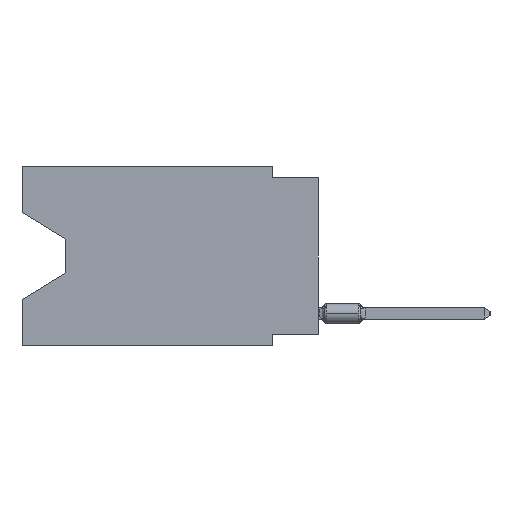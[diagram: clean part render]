
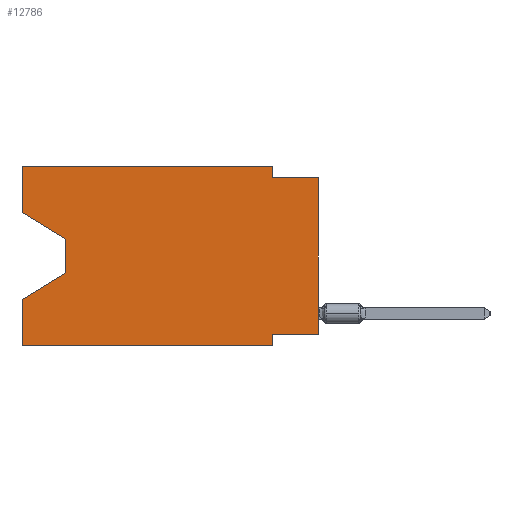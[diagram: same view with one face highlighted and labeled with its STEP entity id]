
A CAD part, left-side view. The second image highlights one B-rep face of the part: STEP entity #12786.
In plain terms, the highlighted planar face has unit normal (-1, 0, 0).
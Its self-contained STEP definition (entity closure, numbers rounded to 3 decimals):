
#658 = CARTESIAN_POINT ( 'NONE',  ( 0., 16.383, -2.546 ) ) ;
#814 = VERTEX_POINT ( 'NONE', #5526 ) ;
#831 = VERTEX_POINT ( 'NONE', #15682 ) ;
#1392 = EDGE_CURVE ( 'NONE', #14095, #26690, #18622, .T. ) ;
#1428 = EDGE_CURVE ( 'NONE', #23156, #831, #18884, .T. ) ;
#1508 = PLANE ( 'NONE',  #12656 ) ;
#3536 = CARTESIAN_POINT ( 'NONE',  ( 0., 2.54, 0. ) ) ;
#4026 = CARTESIAN_POINT ( 'NONE',  ( 0., 16.383, -2.546 ) ) ;
#4365 = ORIENTED_EDGE ( 'NONE', *, *, #9238, .F. ) ;
#4608 = ORIENTED_EDGE ( 'NONE', *, *, #15362, .F. ) ;
#4651 = EDGE_CURVE ( 'NONE', #23824, #18407, #12228, .T. ) ;
#4739 = DIRECTION ( 'NONE',  ( 0., 1., 0. ) ) ;
#4942 = ORIENTED_EDGE ( 'NONE', *, *, #26467, .T. ) ;
#5325 = VECTOR ( 'NONE', #8825, 1000. ) ;
#5526 = CARTESIAN_POINT ( 'NONE',  ( 0., 16.383, -7.36 ) ) ;
#5918 = VECTOR ( 'NONE', #17950, 1000. ) ;
#5922 = EDGE_CURVE ( 'NONE', #18739, #14095, #11374, .T. ) ;
#6978 = DIRECTION ( 'NONE',  ( 0., 0., 1. ) ) ;
#7439 = ORIENTED_EDGE ( 'NONE', *, *, #20495, .F. ) ;
#7623 = VERTEX_POINT ( 'NONE', #8068 ) ;
#8068 = CARTESIAN_POINT ( 'NONE',  ( 0., 16.383, 0. ) ) ;
#8126 = DIRECTION ( 'NONE',  ( 1., 0., 0. ) ) ;
#8310 = CARTESIAN_POINT ( 'NONE',  ( 0., 2.54, -9.906 ) ) ;
#8825 = DIRECTION ( 'NONE',  ( 0., 0., 1. ) ) ;
#9098 = CARTESIAN_POINT ( 'NONE',  ( 0., 16.383, 0. ) ) ;
#9229 = LINE ( 'NONE', #17555, #21300 ) ;
#9238 = EDGE_CURVE ( 'NONE', #18739, #7623, #9229, .T. ) ;
#9372 = VECTOR ( 'NONE', #12106, 1000. ) ;
#9684 = LINE ( 'NONE', #9814, #14362 ) ;
#9814 = CARTESIAN_POINT ( 'NONE',  ( 0., 16.383, 0. ) ) ;
#9944 = ORIENTED_EDGE ( 'NONE', *, *, #1392, .T. ) ;
#10375 = LINE ( 'NONE', #13801, #11232 ) ;
#10435 = EDGE_CURVE ( 'NONE', #20657, #814, #22066, .T. ) ;
#10722 = VECTOR ( 'NONE', #20863, 1000. ) ;
#10753 = VECTOR ( 'NONE', #13007, 1000. ) ;
#10882 = EDGE_CURVE ( 'NONE', #26690, #814, #19649, .T. ) ;
#10990 = VERTEX_POINT ( 'NONE', #11871 ) ;
#11232 = VECTOR ( 'NONE', #22560, 1000. ) ;
#11374 = LINE ( 'NONE', #658, #20936 ) ;
#11871 = CARTESIAN_POINT ( 'NONE',  ( 0., 0., -0.635 ) ) ;
#12106 = DIRECTION ( 'NONE',  ( 0., 0., -1. ) ) ;
#12228 = LINE ( 'NONE', #23520, #15601 ) ;
#12287 = ORIENTED_EDGE ( 'NONE', *, *, #5922, .T. ) ;
#12656 = AXIS2_PLACEMENT_3D ( 'NONE', #18718, #8126, #23221 ) ;
#12786 = ADVANCED_FACE ( 'NONE', ( #20826 ), #1508, .F. ) ;
#13007 = DIRECTION ( 'NONE',  ( 0., 0.855, -0.519 ) ) ;
#13801 = CARTESIAN_POINT ( 'NONE',  ( 0., 0., 0. ) ) ;
#13845 = CARTESIAN_POINT ( 'NONE',  ( 0., 0., -0.635 ) ) ;
#14095 = VERTEX_POINT ( 'NONE', #23508 ) ;
#14334 = ORIENTED_EDGE ( 'NONE', *, *, #14576, .F. ) ;
#14362 = VECTOR ( 'NONE', #16449, 1000. ) ;
#14481 = DIRECTION ( 'NONE',  ( 0., 0., -1. ) ) ;
#14576 = EDGE_CURVE ( 'NONE', #18407, #10990, #15559, .T. ) ;
#15038 = VECTOR ( 'NONE', #25422, 1000. ) ;
#15117 = CARTESIAN_POINT ( 'NONE',  ( 0., 16.383, -9.906 ) ) ;
#15242 = CARTESIAN_POINT ( 'NONE',  ( 0., 16.383, -9.906 ) ) ;
#15362 = EDGE_CURVE ( 'NONE', #7623, #23824, #9684, .T. ) ;
#15559 = LINE ( 'NONE', #13845, #5918 ) ;
#15601 = VECTOR ( 'NONE', #14481, 1000. ) ;
#15682 = CARTESIAN_POINT ( 'NONE',  ( 0., 2.54, -9.906 ) ) ;
#15940 = EDGE_CURVE ( 'NONE', #27013, #10990, #10375, .T. ) ;
#16449 = DIRECTION ( 'NONE',  ( 0., -1., 0. ) ) ;
#17544 = ORIENTED_EDGE ( 'NONE', *, *, #10882, .T. ) ;
#17555 = CARTESIAN_POINT ( 'NONE',  ( 0., 16.383, 0. ) ) ;
#17819 = ORIENTED_EDGE ( 'NONE', *, *, #15940, .T. ) ;
#17860 = LINE ( 'NONE', #22239, #22038 ) ;
#17950 = DIRECTION ( 'NONE',  ( 0., -1., 0. ) ) ;
#18407 = VERTEX_POINT ( 'NONE', #23980 ) ;
#18559 = LINE ( 'NONE', #15242, #15038 ) ;
#18622 = LINE ( 'NONE', #24958, #10722 ) ;
#18718 = CARTESIAN_POINT ( 'NONE',  ( 0., 16.383, 0. ) ) ;
#18739 = VERTEX_POINT ( 'NONE', #4026 ) ;
#18884 = LINE ( 'NONE', #8310, #9372 ) ;
#19649 = LINE ( 'NONE', #22031, #10753 ) ;
#20495 = EDGE_CURVE ( 'NONE', #27013, #23156, #17860, .T. ) ;
#20657 = VERTEX_POINT ( 'NONE', #15117 ) ;
#20825 = CARTESIAN_POINT ( 'NONE',  ( 0., 0., -9.271 ) ) ;
#20826 = FACE_OUTER_BOUND ( 'NONE', #27773, .T. ) ;
#20863 = DIRECTION ( 'NONE',  ( 0., 0., -1. ) ) ;
#20892 = ORIENTED_EDGE ( 'NONE', *, *, #10435, .F. ) ;
#20936 = VECTOR ( 'NONE', #23663, 1000. ) ;
#21300 = VECTOR ( 'NONE', #6978, 1000. ) ;
#21497 = ORIENTED_EDGE ( 'NONE', *, *, #1428, .F. ) ;
#21838 = CARTESIAN_POINT ( 'NONE',  ( 0., 13.97, -5.893 ) ) ;
#22031 = CARTESIAN_POINT ( 'NONE',  ( 0., 13.97, -5.893 ) ) ;
#22038 = VECTOR ( 'NONE', #4739, 1000. ) ;
#22066 = LINE ( 'NONE', #9098, #5325 ) ;
#22239 = CARTESIAN_POINT ( 'NONE',  ( 0., 0., -9.271 ) ) ;
#22560 = DIRECTION ( 'NONE',  ( 0., 0., 1. ) ) ;
#23156 = VERTEX_POINT ( 'NONE', #27588 ) ;
#23221 = DIRECTION ( 'NONE',  ( 0., 0., -1. ) ) ;
#23508 = CARTESIAN_POINT ( 'NONE',  ( 0., 13.97, -4.013 ) ) ;
#23520 = CARTESIAN_POINT ( 'NONE',  ( 0., 2.54, 0. ) ) ;
#23663 = DIRECTION ( 'NONE',  ( 0., -0.855, -0.519 ) ) ;
#23824 = VERTEX_POINT ( 'NONE', #3536 ) ;
#23980 = CARTESIAN_POINT ( 'NONE',  ( 0., 2.54, -0.635 ) ) ;
#24958 = CARTESIAN_POINT ( 'NONE',  ( 0., 13.97, -4.013 ) ) ;
#25422 = DIRECTION ( 'NONE',  ( 0., -1., 0. ) ) ;
#25829 = ORIENTED_EDGE ( 'NONE', *, *, #4651, .F. ) ;
#26467 = EDGE_CURVE ( 'NONE', #20657, #831, #18559, .T. ) ;
#26690 = VERTEX_POINT ( 'NONE', #21838 ) ;
#27013 = VERTEX_POINT ( 'NONE', #20825 ) ;
#27588 = CARTESIAN_POINT ( 'NONE',  ( 0., 2.54, -9.271 ) ) ;
#27773 = EDGE_LOOP ( 'NONE', ( #12287, #9944, #17544, #20892, #4942, #21497, #7439, #17819, #14334, #25829, #4608, #4365 ) ) ;
